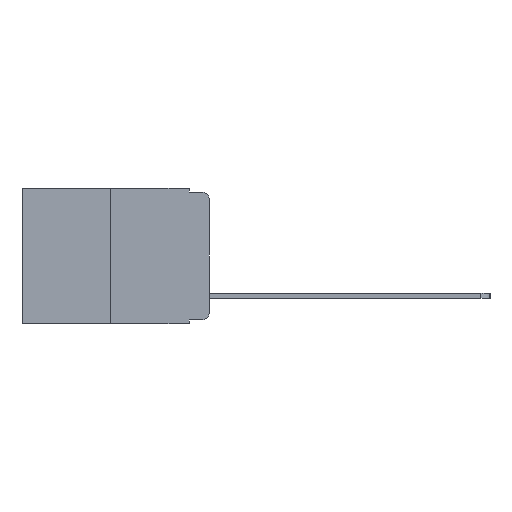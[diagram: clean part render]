
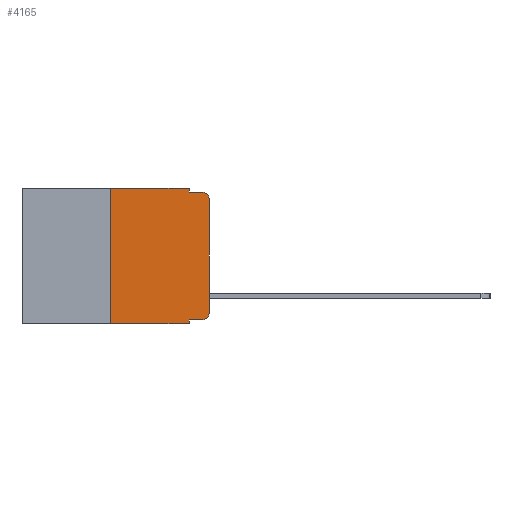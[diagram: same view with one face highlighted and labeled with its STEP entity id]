
A CAD part, left-side view. The second image highlights one B-rep face of the part: STEP entity #4165.
In plain terms, the highlighted planar face has unit normal (-1, 0, 0).
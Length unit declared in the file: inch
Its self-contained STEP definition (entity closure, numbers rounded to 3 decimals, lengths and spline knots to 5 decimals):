
#48 = CARTESIAN_POINT ( 'NONE',  ( 0., 0., 0. ) ) ;
#201 = EDGE_CURVE ( 'NONE', #8446, #4712, #5147, .T. ) ;
#411 = DIRECTION ( 'NONE',  ( -1., 0., 0. ) ) ;
#694 = VECTOR ( 'NONE', #10797, 39.37008 ) ;
#800 = ORIENTED_EDGE ( 'NONE', *, *, #15314, .F. ) ;
#804 = VECTOR ( 'NONE', #16078, 39.37008 ) ;
#1119 = VECTOR ( 'NONE', #16119, 39.37008 ) ;
#1703 = DIRECTION ( 'NONE',  ( 0., 0., -1. ) ) ;
#1804 = VERTEX_POINT ( 'NONE', #14383 ) ;
#2081 = CIRCLE ( 'NONE', #7409, 0.02 ) ;
#2310 = EDGE_CURVE ( 'NONE', #10492, #4712, #11054, .T. ) ;
#2466 = CIRCLE ( 'NONE', #15592, 0.02 ) ;
#3133 = LINE ( 'NONE', #4438, #5862 ) ;
#3752 = DIRECTION ( 'NONE',  ( 0., 0., -1. ) ) ;
#3951 = VECTOR ( 'NONE', #15360, 39.37008 ) ;
#4165 = ADVANCED_FACE ( 'NONE', ( #6341 ), #8652, .F. ) ;
#4355 = LINE ( 'NONE', #48, #694 ) ;
#4438 = CARTESIAN_POINT ( 'NONE',  ( 0., 0.473, 0. ) ) ;
#4682 = AXIS2_PLACEMENT_3D ( 'NONE', #13978, #8896, #3752 ) ;
#4712 = VERTEX_POINT ( 'NONE', #7116 ) ;
#5147 = LINE ( 'NONE', #11526, #11301 ) ;
#5303 = DIRECTION ( 'NONE',  ( -1., 0., 0. ) ) ;
#5385 = CARTESIAN_POINT ( 'NONE',  ( 0., 0., -0.313 ) ) ;
#5586 = LINE ( 'NONE', #12514, #1119 ) ;
#5862 = VECTOR ( 'NONE', #9787, 39.37008 ) ;
#6015 = CARTESIAN_POINT ( 'NONE',  ( 0., 0.473, -0.343 ) ) ;
#6147 = ORIENTED_EDGE ( 'NONE', *, *, #14585, .T. ) ;
#6218 = EDGE_CURVE ( 'NONE', #10492, #6252, #16276, .T. ) ;
#6252 = VERTEX_POINT ( 'NONE', #14926 ) ;
#6341 = FACE_OUTER_BOUND ( 'NONE', #14046, .T. ) ;
#6385 = ORIENTED_EDGE ( 'NONE', *, *, #11757, .T. ) ;
#6541 = CARTESIAN_POINT ( 'NONE',  ( 0., 0.051, -0.01 ) ) ;
#6617 = ORIENTED_EDGE ( 'NONE', *, *, #2310, .T. ) ;
#6844 = ORIENTED_EDGE ( 'NONE', *, *, #9243, .T. ) ;
#7026 = ORIENTED_EDGE ( 'NONE', *, *, #13913, .F. ) ;
#7116 = CARTESIAN_POINT ( 'NONE',  ( 0., 0.051, -0.343 ) ) ;
#7179 = CARTESIAN_POINT ( 'NONE',  ( 0., 0.02, -0.01 ) ) ;
#7285 = ORIENTED_EDGE ( 'NONE', *, *, #201, .F. ) ;
#7304 = VERTEX_POINT ( 'NONE', #12390 ) ;
#7391 = LINE ( 'NONE', #8918, #10871 ) ;
#7409 = AXIS2_PLACEMENT_3D ( 'NONE', #13043, #5303, #14265 ) ;
#7596 = ORIENTED_EDGE ( 'NONE', *, *, #14945, .T. ) ;
#8446 = VERTEX_POINT ( 'NONE', #14842 ) ;
#8481 = CARTESIAN_POINT ( 'NONE',  ( 0., 0.02, -0.03 ) ) ;
#8652 = PLANE ( 'NONE',  #4682 ) ;
#8896 = DIRECTION ( 'NONE',  ( 1., 0., 0. ) ) ;
#8918 = CARTESIAN_POINT ( 'NONE',  ( 0., 0.051, -0.333 ) ) ;
#9243 = EDGE_CURVE ( 'NONE', #12613, #1804, #4355, .T. ) ;
#9385 = VERTEX_POINT ( 'NONE', #7179 ) ;
#9787 = DIRECTION ( 'NONE',  ( 0., -1., 0. ) ) ;
#9845 = DIRECTION ( 'NONE',  ( 0., 0., -1. ) ) ;
#10259 = DIRECTION ( 'NONE',  ( 0., -1., 0. ) ) ;
#10492 = VERTEX_POINT ( 'NONE', #16411 ) ;
#10797 = DIRECTION ( 'NONE',  ( 0., 0., 1. ) ) ;
#10871 = VECTOR ( 'NONE', #10259, 39.37008 ) ;
#11054 = LINE ( 'NONE', #6015, #804 ) ;
#11117 = ORIENTED_EDGE ( 'NONE', *, *, #14882, .F. ) ;
#11259 = ORIENTED_EDGE ( 'NONE', *, *, #6218, .F. ) ;
#11301 = VECTOR ( 'NONE', #1703, 39.37008 ) ;
#11526 = CARTESIAN_POINT ( 'NONE',  ( 0., 0.051, 0. ) ) ;
#11757 = EDGE_CURVE ( 'NONE', #8446, #12106, #7391, .T. ) ;
#11895 = VERTEX_POINT ( 'NONE', #15562 ) ;
#12106 = VERTEX_POINT ( 'NONE', #12297 ) ;
#12297 = CARTESIAN_POINT ( 'NONE',  ( 0., 0.02, -0.333 ) ) ;
#12390 = CARTESIAN_POINT ( 'NONE',  ( 0., 0.051, 0. ) ) ;
#12514 = CARTESIAN_POINT ( 'NONE',  ( 0., 0.051, 0. ) ) ;
#12613 = VERTEX_POINT ( 'NONE', #5385 ) ;
#13043 = CARTESIAN_POINT ( 'NONE',  ( 0., 0.02, -0.313 ) ) ;
#13845 = LINE ( 'NONE', #6541, #3951 ) ;
#13913 = EDGE_CURVE ( 'NONE', #6252, #7304, #3133, .T. ) ;
#13978 = CARTESIAN_POINT ( 'NONE',  ( 0., 0.473, 0. ) ) ;
#14046 = EDGE_LOOP ( 'NONE', ( #6844, #6147, #11117, #800, #7026, #11259, #6617, #7285, #6385, #7596 ) ) ;
#14265 = DIRECTION ( 'NONE',  ( 0., 0., -1. ) ) ;
#14383 = CARTESIAN_POINT ( 'NONE',  ( 0., 0., -0.03 ) ) ;
#14585 = EDGE_CURVE ( 'NONE', #1804, #9385, #2466, .T. ) ;
#14842 = CARTESIAN_POINT ( 'NONE',  ( 0., 0.051, -0.333 ) ) ;
#14878 = CARTESIAN_POINT ( 'NONE',  ( 0., 0.25, 0. ) ) ;
#14882 = EDGE_CURVE ( 'NONE', #11895, #9385, #13845, .T. ) ;
#14926 = CARTESIAN_POINT ( 'NONE',  ( 0., 0.25, 0. ) ) ;
#14945 = EDGE_CURVE ( 'NONE', #12106, #12613, #2081, .T. ) ;
#15314 = EDGE_CURVE ( 'NONE', #7304, #11895, #5586, .T. ) ;
#15360 = DIRECTION ( 'NONE',  ( 0., -1., 0. ) ) ;
#15417 = DIRECTION ( 'NONE',  ( 0., 0., 1. ) ) ;
#15562 = CARTESIAN_POINT ( 'NONE',  ( 0., 0.051, -0.01 ) ) ;
#15592 = AXIS2_PLACEMENT_3D ( 'NONE', #8481, #411, #9845 ) ;
#15909 = VECTOR ( 'NONE', #15417, 39.37008 ) ;
#16078 = DIRECTION ( 'NONE',  ( 0., -1., 0. ) ) ;
#16119 = DIRECTION ( 'NONE',  ( 0., 0., -1. ) ) ;
#16276 = LINE ( 'NONE', #14878, #15909 ) ;
#16411 = CARTESIAN_POINT ( 'NONE',  ( 0., 0.25, -0.343 ) ) ;
